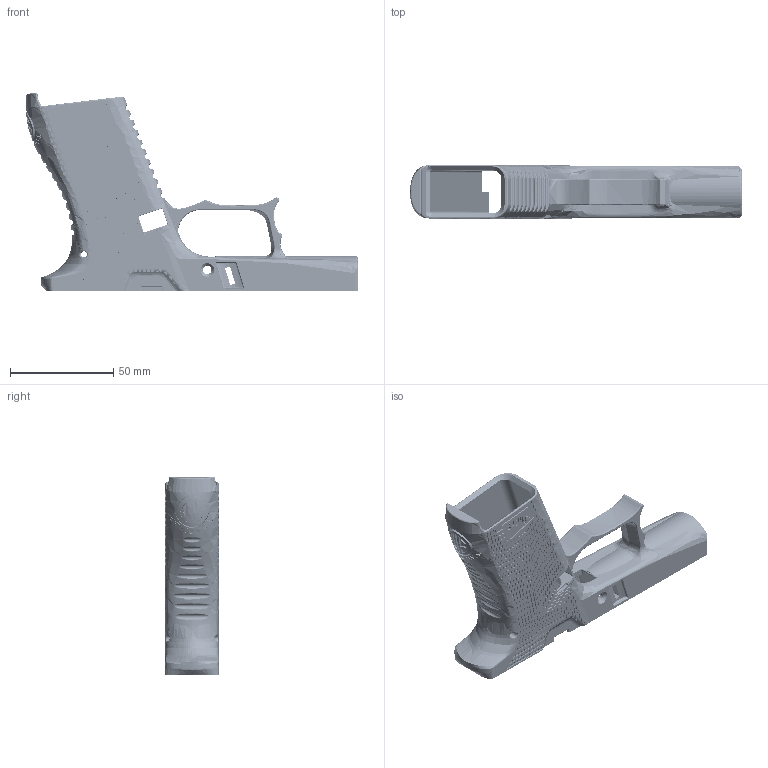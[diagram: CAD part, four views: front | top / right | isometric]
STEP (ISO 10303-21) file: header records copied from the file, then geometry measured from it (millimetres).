
FILE_DESCRIPTION (( 'STEP AP203' ), '1' );
FILE_NAME ('43X SnakeSkin FDM.STEP', '2020-12-17T01:17:36', ( '' ), ( '' ), 'SwSTEP 2.0', 'SolidWorks 2016', '' );
FILE_SCHEMA (( 'CONFIG_CONTROL_DESIGN' ));
Products named in the file (1): 43X SnakeSkin FDM
Bounding box: 160.56 x 25.9 x 95.92 mm (x, y, z)
Volume: 62752.7 mm3; surface area: 42286.6 mm2
Topology: 1 solids, 1 shells, 8065 faces, 20764 edges, 13701 vertices
Faces by surface type: plane 2922, bspline 2590, cylinder 2513, torus 26, cone 12, sphere 2
Entity records: 399617 total; most frequent: CARTESIAN_POINT 228338, ORIENTED_EDGE 41456, DIRECTION 24369, EDGE_CURVE 20728, VERTEX_POINT 13701, B_SPLINE_CURVE_WITH_KNOTS 9850, EDGE_LOOP 9123, LINE 8125
